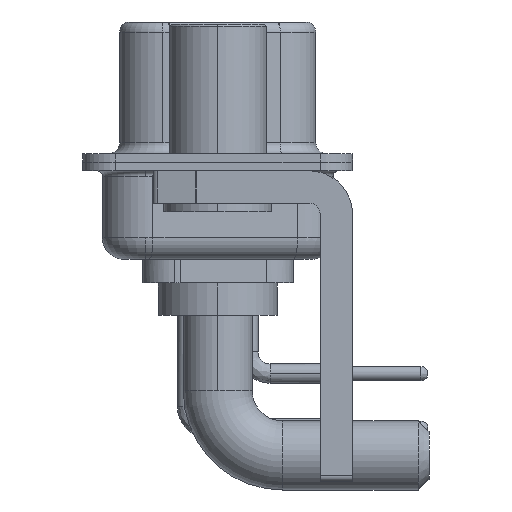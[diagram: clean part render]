
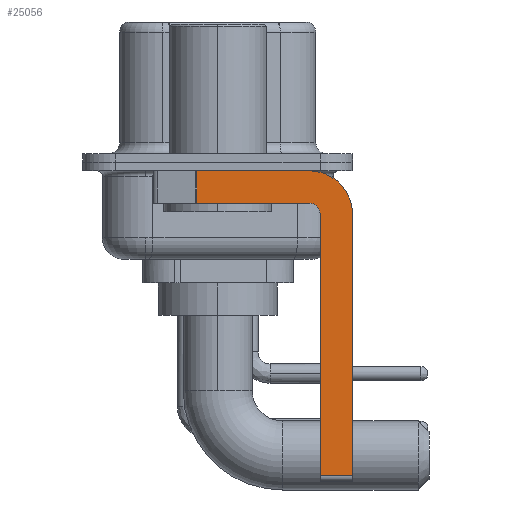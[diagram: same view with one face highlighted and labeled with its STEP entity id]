
A CAD part, left-side view. The second image highlights one B-rep face of the part: STEP entity #25056.
In plain terms, the highlighted planar face has unit normal (-1, 0, 0).
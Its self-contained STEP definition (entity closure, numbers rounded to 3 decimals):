
#203 = LINE ( 'NONE', #13533, #16504 ) ;
#745 = CARTESIAN_POINT ( 'NONE',  ( -2.9, -4.25, -2.4 ) ) ;
#1449 = EDGE_LOOP ( 'NONE', ( #9443, #14071, #17523, #15327, #11726, #27941, #9604, #9680 ) ) ;
#1958 = VERTEX_POINT ( 'NONE', #15217 ) ;
#2835 = PLANE ( 'NONE',  #8821 ) ;
#2966 = FACE_OUTER_BOUND ( 'NONE', #1449, .T. ) ;
#3029 = VECTOR ( 'NONE', #23442, 1000. ) ;
#3114 = DIRECTION ( 'NONE',  ( 0., 0., -1. ) ) ;
#3590 = VERTEX_POINT ( 'NONE', #15933 ) ;
#4084 = CIRCLE ( 'NONE', #18779, 2. ) ;
#4637 = EDGE_CURVE ( 'NONE', #8632, #16514, #4084, .T. ) ;
#5053 = VERTEX_POINT ( 'NONE', #27815 ) ;
#5194 = CARTESIAN_POINT ( 'NONE',  ( -2.9, -4.25, -2.4 ) ) ;
#5462 = DIRECTION ( 'NONE',  ( 0., 0., -1. ) ) ;
#5510 = AXIS2_PLACEMENT_3D ( 'NONE', #5194, #18681, #18541 ) ;
#5648 = CARTESIAN_POINT ( 'NONE',  ( -2.9, -4.25, -14.55 ) ) ;
#5678 = DIRECTION ( 'NONE',  ( 0., 0., -1. ) ) ;
#5810 = CARTESIAN_POINT ( 'NONE',  ( -2.9, -6.25, -2.4 ) ) ;
#6617 = LINE ( 'NONE', #8994, #19549 ) ;
#6849 = DIRECTION ( 'NONE',  ( 0., -1., 0. ) ) ;
#7727 = CARTESIAN_POINT ( 'NONE',  ( -2.9, -4.25, -0.4 ) ) ;
#8632 = VERTEX_POINT ( 'NONE', #7727 ) ;
#8821 = AXIS2_PLACEMENT_3D ( 'NONE', #745, #27706, #3114 ) ;
#8994 = CARTESIAN_POINT ( 'NONE',  ( -2.9, 0.978, -1.9 ) ) ;
#9443 = ORIENTED_EDGE ( 'NONE', *, *, #26847, .F. ) ;
#9464 = VERTEX_POINT ( 'NONE', #21429 ) ;
#9604 = ORIENTED_EDGE ( 'NONE', *, *, #16137, .F. ) ;
#9680 = ORIENTED_EDGE ( 'NONE', *, *, #4637, .F. ) ;
#10436 = DIRECTION ( 'NONE',  ( 0., 0., 1. ) ) ;
#11726 = ORIENTED_EDGE ( 'NONE', *, *, #13274, .F. ) ;
#11865 = CARTESIAN_POINT ( 'NONE',  ( -2.9, -4.25, -1.9 ) ) ;
#12166 = DIRECTION ( 'NONE',  ( 0., -1., 0. ) ) ;
#12669 = LINE ( 'NONE', #17267, #25428 ) ;
#12811 = VECTOR ( 'NONE', #5678, 1000. ) ;
#13274 = EDGE_CURVE ( 'NONE', #3590, #13623, #12669, .T. ) ;
#13533 = CARTESIAN_POINT ( 'NONE',  ( -2.9, 3., -0.4 ) ) ;
#13623 = VERTEX_POINT ( 'NONE', #27756 ) ;
#14071 = ORIENTED_EDGE ( 'NONE', *, *, #17455, .T. ) ;
#15217 = CARTESIAN_POINT ( 'NONE',  ( -2.9, 0.978, -0.4 ) ) ;
#15327 = ORIENTED_EDGE ( 'NONE', *, *, #25013, .F. ) ;
#15933 = CARTESIAN_POINT ( 'NONE',  ( -2.9, -4.75, -14.55 ) ) ;
#16137 = EDGE_CURVE ( 'NONE', #16514, #5053, #18904, .T. ) ;
#16321 = LINE ( 'NONE', #11865, #3029 ) ;
#16504 = VECTOR ( 'NONE', #6849, 1000. ) ;
#16514 = VERTEX_POINT ( 'NONE', #20220 ) ;
#16599 = CARTESIAN_POINT ( 'NONE',  ( -2.9, -4.25, -2.4 ) ) ;
#16645 = EDGE_CURVE ( 'NONE', #3590, #5053, #21521, .T. ) ;
#17267 = CARTESIAN_POINT ( 'NONE',  ( -2.9, -4.75, -14.8 ) ) ;
#17455 = EDGE_CURVE ( 'NONE', #1958, #9464, #6617, .T. ) ;
#17523 = ORIENTED_EDGE ( 'NONE', *, *, #20864, .F. ) ;
#18192 = DIRECTION ( 'NONE',  ( 0., 0., -1. ) ) ;
#18537 = CARTESIAN_POINT ( 'NONE',  ( -2.9, -4.25, -1.9 ) ) ;
#18541 = DIRECTION ( 'NONE',  ( 0., 0., 1. ) ) ;
#18681 = DIRECTION ( 'NONE',  ( -1., 0., 0. ) ) ;
#18779 = AXIS2_PLACEMENT_3D ( 'NONE', #16599, #25640, #5462 ) ;
#18787 = CIRCLE ( 'NONE', #5510, 0.5 ) ;
#18904 = LINE ( 'NONE', #5810, #12811 ) ;
#19512 = VECTOR ( 'NONE', #12166, 1000. ) ;
#19549 = VECTOR ( 'NONE', #18192, 1000. ) ;
#20220 = CARTESIAN_POINT ( 'NONE',  ( -2.9, -6.25, -2.4 ) ) ;
#20864 = EDGE_CURVE ( 'NONE', #23643, #9464, #16321, .T. ) ;
#21429 = CARTESIAN_POINT ( 'NONE',  ( -2.9, 0.978, -1.9 ) ) ;
#21521 = LINE ( 'NONE', #5648, #19512 ) ;
#23442 = DIRECTION ( 'NONE',  ( 0., 1., 0. ) ) ;
#23643 = VERTEX_POINT ( 'NONE', #18537 ) ;
#25013 = EDGE_CURVE ( 'NONE', #13623, #23643, #18787, .T. ) ;
#25056 = ADVANCED_FACE ( 'NONE', ( #2966 ), #2835, .F. ) ;
#25428 = VECTOR ( 'NONE', #10436, 1000. ) ;
#25640 = DIRECTION ( 'NONE',  ( 1., 0., 0. ) ) ;
#26847 = EDGE_CURVE ( 'NONE', #1958, #8632, #203, .T. ) ;
#27706 = DIRECTION ( 'NONE',  ( 1., 0., 0. ) ) ;
#27756 = CARTESIAN_POINT ( 'NONE',  ( -2.9, -4.75, -2.4 ) ) ;
#27815 = CARTESIAN_POINT ( 'NONE',  ( -2.9, -6.25, -14.55 ) ) ;
#27941 = ORIENTED_EDGE ( 'NONE', *, *, #16645, .T. ) ;
